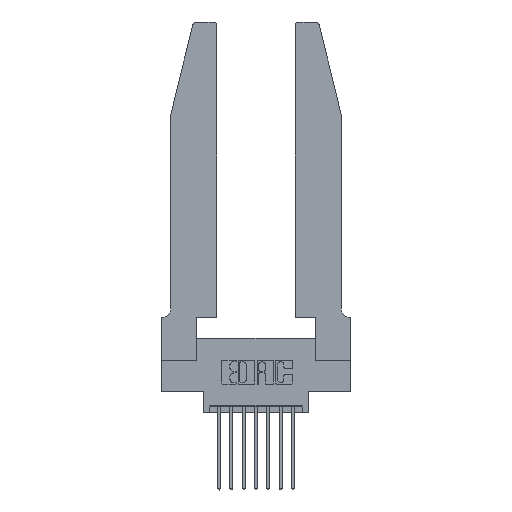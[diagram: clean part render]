
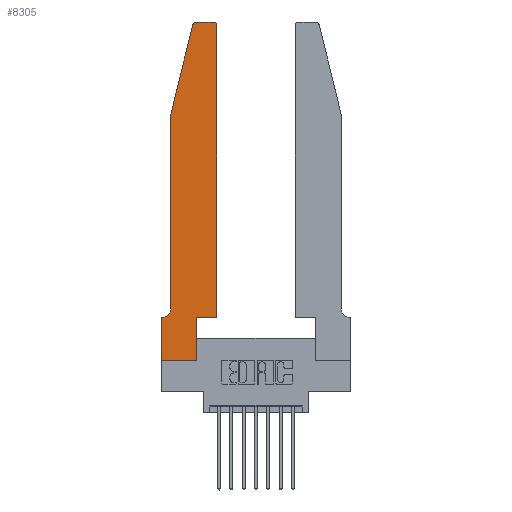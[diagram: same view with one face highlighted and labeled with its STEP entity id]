
A CAD part, top view. The second image highlights one B-rep face of the part: STEP entity #8305.
In plain terms, the highlighted planar face has unit normal (0, 0, 1).
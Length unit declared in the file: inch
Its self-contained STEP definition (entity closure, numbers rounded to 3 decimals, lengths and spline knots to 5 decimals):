
#348 = DIRECTION ( 'NONE',  ( 1., 0., 0. ) ) ;
#450 = LINE ( 'NONE', #12811, #12713 ) ;
#699 = VECTOR ( 'NONE', #12387, 39.37008 ) ;
#702 = VERTEX_POINT ( 'NONE', #7912 ) ;
#736 = EDGE_CURVE ( 'NONE', #7802, #9223, #2935, .T. ) ;
#1038 = DIRECTION ( 'NONE',  ( 0., 0., -1. ) ) ;
#1045 = CARTESIAN_POINT ( 'NONE',  ( 0.0755, 0.42, 0.37 ) ) ;
#1303 = CARTESIAN_POINT ( 'NONE',  ( 0.0055, 0.35, 0.37 ) ) ;
#1394 = CARTESIAN_POINT ( 'NONE',  ( 0.0755, 2., 0.37 ) ) ;
#1478 = AXIS2_PLACEMENT_3D ( 'NONE', #13972, #9352, #8175 ) ;
#1510 = VERTEX_POINT ( 'NONE', #6404 ) ;
#1597 = VERTEX_POINT ( 'NONE', #14766 ) ;
#1685 = ORIENTED_EDGE ( 'NONE', *, *, #6427, .T. ) ;
#1969 = ORIENTED_EDGE ( 'NONE', *, *, #7884, .T. ) ;
#2145 = CARTESIAN_POINT ( 'NONE',  ( 0.2865, 0., 0.37 ) ) ;
#2221 = DIRECTION ( 'NONE',  ( -1., 0., 0. ) ) ;
#2260 = VECTOR ( 'NONE', #5766, 39.37008 ) ;
#2399 = VERTEX_POINT ( 'NONE', #1045 ) ;
#2402 = PLANE ( 'NONE',  #1478 ) ;
#2427 = EDGE_CURVE ( 'NONE', #6541, #8935, #13926, .T. ) ;
#2564 = VECTOR ( 'NONE', #5224, 39.37008 ) ;
#2668 = CARTESIAN_POINT ( 'NONE',  ( 0.2605, 2.75, 0.37 ) ) ;
#2935 = LINE ( 'NONE', #11132, #2564 ) ;
#3100 = LINE ( 'NONE', #3398, #11329 ) ;
#3398 = CARTESIAN_POINT ( 'NONE',  ( 0., 0., 0.37 ) ) ;
#3445 = CARTESIAN_POINT ( 'NONE',  ( 0.2865, 0.35, 0.37 ) ) ;
#3458 = ORIENTED_EDGE ( 'NONE', *, *, #5617, .T. ) ;
#3459 = CARTESIAN_POINT ( 'NONE',  ( 0., 0., 0.37 ) ) ;
#3546 = ORIENTED_EDGE ( 'NONE', *, *, #7677, .T. ) ;
#3768 = EDGE_CURVE ( 'NONE', #702, #1597, #13192, .T. ) ;
#3848 = VERTEX_POINT ( 'NONE', #2145 ) ;
#4008 = CARTESIAN_POINT ( 'NONE',  ( 0.4505, 0.35, 0.37 ) ) ;
#4120 = LINE ( 'NONE', #8700, #2260 ) ;
#4669 = VECTOR ( 'NONE', #5792, 39.37008 ) ;
#4686 = CIRCLE ( 'NONE', #7232, 0.03 ) ;
#5182 = ORIENTED_EDGE ( 'NONE', *, *, #14514, .T. ) ;
#5224 = DIRECTION ( 'NONE',  ( -0.239, -0.971, 0. ) ) ;
#5379 = EDGE_LOOP ( 'NONE', ( #5735, #5182, #12757, #12545, #8668, #9898, #7808, #5740, #3546, #1685, #1969, #3458 ) ) ;
#5617 = EDGE_CURVE ( 'NONE', #14683, #702, #8223, .T. ) ;
#5735 = ORIENTED_EDGE ( 'NONE', *, *, #3768, .T. ) ;
#5740 = ORIENTED_EDGE ( 'NONE', *, *, #10957, .T. ) ;
#5766 = DIRECTION ( 'NONE',  ( 0., -1., 0. ) ) ;
#5792 = DIRECTION ( 'NONE',  ( 0., -1., 0. ) ) ;
#6404 = CARTESIAN_POINT ( 'NONE',  ( 0.4505, 0.35, 0.37 ) ) ;
#6427 = EDGE_CURVE ( 'NONE', #7711, #1510, #14573, .T. ) ;
#6541 = VERTEX_POINT ( 'NONE', #14505 ) ;
#6620 = EDGE_CURVE ( 'NONE', #2399, #13671, #14744, .T. ) ;
#6941 = DIRECTION ( 'NONE',  ( 0., 1., 0. ) ) ;
#7044 = DIRECTION ( 'NONE',  ( 1., 0., 0. ) ) ;
#7232 = AXIS2_PLACEMENT_3D ( 'NONE', #10941, #13124, #348 ) ;
#7248 = CARTESIAN_POINT ( 'NONE',  ( 0.2865, 0.35, 0.37 ) ) ;
#7457 = VECTOR ( 'NONE', #7636, 39.37008 ) ;
#7523 = AXIS2_PLACEMENT_3D ( 'NONE', #12175, #13338, #14239 ) ;
#7573 = CARTESIAN_POINT ( 'NONE',  ( 0.4505, 2.72, 0.37 ) ) ;
#7636 = DIRECTION ( 'NONE',  ( 0., 1., 0. ) ) ;
#7640 = VECTOR ( 'NONE', #6941, 39.37008 ) ;
#7677 = EDGE_CURVE ( 'NONE', #3848, #7711, #9638, .T. ) ;
#7711 = VERTEX_POINT ( 'NONE', #7248 ) ;
#7802 = VERTEX_POINT ( 'NONE', #8090 ) ;
#7808 = ORIENTED_EDGE ( 'NONE', *, *, #2427, .T. ) ;
#7884 = EDGE_CURVE ( 'NONE', #1510, #14683, #13808, .T. ) ;
#7912 = CARTESIAN_POINT ( 'NONE',  ( 0.4205, 2.75, 0.37 ) ) ;
#7931 = CARTESIAN_POINT ( 'NONE',  ( 0.4505, 0.35, 0.37 ) ) ;
#8077 = EDGE_CURVE ( 'NONE', #9223, #2399, #4120, .T. ) ;
#8090 = CARTESIAN_POINT ( 'NONE',  ( 0.25487, 2.72718, 0.37 ) ) ;
#8175 = DIRECTION ( 'NONE',  ( 1., 0., 0. ) ) ;
#8223 = CIRCLE ( 'NONE', #7523, 0.03 ) ;
#8305 = ADVANCED_FACE ( 'NONE', ( #14288 ), #2402, .T. ) ;
#8668 = ORIENTED_EDGE ( 'NONE', *, *, #6620, .T. ) ;
#8700 = CARTESIAN_POINT ( 'NONE',  ( 0.0755, 2., 0.37 ) ) ;
#8811 = VECTOR ( 'NONE', #9917, 39.37008 ) ;
#8935 = VERTEX_POINT ( 'NONE', #10112 ) ;
#9223 = VERTEX_POINT ( 'NONE', #1394 ) ;
#9352 = DIRECTION ( 'NONE',  ( 0., 0., 1. ) ) ;
#9638 = LINE ( 'NONE', #3445, #7640 ) ;
#9898 = ORIENTED_EDGE ( 'NONE', *, *, #13453, .T. ) ;
#9917 = DIRECTION ( 'NONE',  ( -1., 0., 0. ) ) ;
#10112 = CARTESIAN_POINT ( 'NONE',  ( 0., 0., 0.37 ) ) ;
#10941 = CARTESIAN_POINT ( 'NONE',  ( 0.284, 2.72, 0.37 ) ) ;
#10957 = EDGE_CURVE ( 'NONE', #8935, #3848, #3100, .T. ) ;
#11021 = AXIS2_PLACEMENT_3D ( 'NONE', #15017, #1038, #2221 ) ;
#11132 = CARTESIAN_POINT ( 'NONE',  ( 0.0755, 2., 0.37 ) ) ;
#11329 = VECTOR ( 'NONE', #7044, 39.37008 ) ;
#12175 = CARTESIAN_POINT ( 'NONE',  ( 0.4205, 2.72, 0.37 ) ) ;
#12387 = DIRECTION ( 'NONE',  ( 1., 0., 0. ) ) ;
#12545 = ORIENTED_EDGE ( 'NONE', *, *, #8077, .T. ) ;
#12713 = VECTOR ( 'NONE', #13887, 39.37008 ) ;
#12757 = ORIENTED_EDGE ( 'NONE', *, *, #736, .T. ) ;
#12811 = CARTESIAN_POINT ( 'NONE',  ( 0.0755, 0.35, 0.37 ) ) ;
#13124 = DIRECTION ( 'NONE',  ( 0., 0., 1. ) ) ;
#13192 = LINE ( 'NONE', #2668, #8811 ) ;
#13338 = DIRECTION ( 'NONE',  ( 0., 0., 1. ) ) ;
#13453 = EDGE_CURVE ( 'NONE', #13671, #6541, #450, .T. ) ;
#13671 = VERTEX_POINT ( 'NONE', #1303 ) ;
#13808 = LINE ( 'NONE', #4008, #7457 ) ;
#13887 = DIRECTION ( 'NONE',  ( -1., 0., 0. ) ) ;
#13926 = LINE ( 'NONE', #3459, #4669 ) ;
#13972 = CARTESIAN_POINT ( 'NONE',  ( 0., 0.35, 0.37 ) ) ;
#14239 = DIRECTION ( 'NONE',  ( 1., 0., 0. ) ) ;
#14288 = FACE_OUTER_BOUND ( 'NONE', #5379, .T. ) ;
#14505 = CARTESIAN_POINT ( 'NONE',  ( 0., 0.35, 0.37 ) ) ;
#14514 = EDGE_CURVE ( 'NONE', #1597, #7802, #4686, .T. ) ;
#14573 = LINE ( 'NONE', #7931, #699 ) ;
#14683 = VERTEX_POINT ( 'NONE', #7573 ) ;
#14744 = CIRCLE ( 'NONE', #11021, 0.07 ) ;
#14766 = CARTESIAN_POINT ( 'NONE',  ( 0.284, 2.75, 0.37 ) ) ;
#15017 = CARTESIAN_POINT ( 'NONE',  ( 0.0055, 0.42, 0.37 ) ) ;
